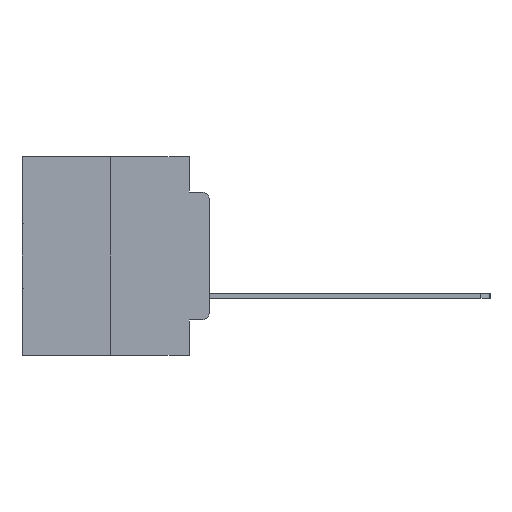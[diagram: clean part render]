
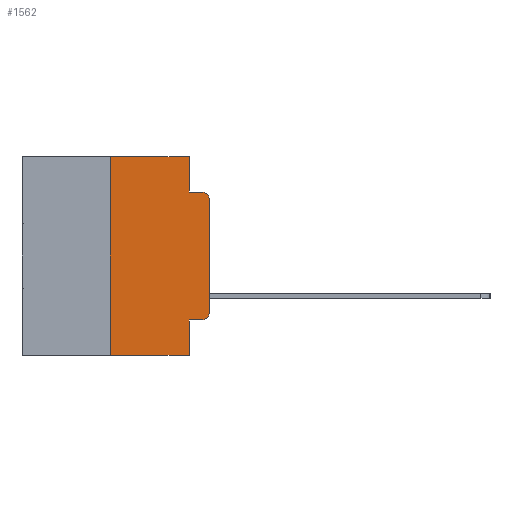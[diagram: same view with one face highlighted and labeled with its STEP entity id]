
A CAD part, left-side view. The second image highlights one B-rep face of the part: STEP entity #1562.
In plain terms, the highlighted planar face has unit normal (-1, 0, 0).
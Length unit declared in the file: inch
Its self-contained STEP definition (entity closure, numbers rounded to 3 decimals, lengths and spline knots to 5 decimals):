
#157 = VERTEX_POINT ( 'NONE', #6908 ) ;
#313 = CARTESIAN_POINT ( 'NONE',  ( 0., 0.473, 0. ) ) ;
#1015 = DIRECTION ( 'NONE',  ( -1., 0., 0. ) ) ;
#1311 = EDGE_CURVE ( 'NONE', #157, #25976, #9049, .T. ) ;
#1342 = ORIENTED_EDGE ( 'NONE', *, *, #24308, .F. ) ;
#1346 = EDGE_LOOP ( 'NONE', ( #4672, #28072, #5410, #11544, #18711, #1342, #20058, #2801, #9098, #3564 ) ) ;
#1423 = VECTOR ( 'NONE', #27654, 39.37008 ) ;
#1562 = ADVANCED_FACE ( 'NONE', ( #13211 ), #24217, .F. ) ;
#1711 = VECTOR ( 'NONE', #5330, 39.37008 ) ;
#1929 = DIRECTION ( 'NONE',  ( 0., 0., -1. ) ) ;
#2098 = CARTESIAN_POINT ( 'NONE',  ( 0., 0.25, 0. ) ) ;
#2108 = DIRECTION ( 'NONE',  ( 0., 0., -1. ) ) ;
#2547 = CARTESIAN_POINT ( 'NONE',  ( 0., 0., 0. ) ) ;
#2667 = VERTEX_POINT ( 'NONE', #3909 ) ;
#2801 = ORIENTED_EDGE ( 'NONE', *, *, #21455, .F. ) ;
#2845 = VECTOR ( 'NONE', #22708, 39.37008 ) ;
#2879 = EDGE_CURVE ( 'NONE', #5140, #157, #10006, .T. ) ;
#2929 = CARTESIAN_POINT ( 'NONE',  ( 0., 0.051, 0. ) ) ;
#3564 = ORIENTED_EDGE ( 'NONE', *, *, #17172, .T. ) ;
#3574 = CARTESIAN_POINT ( 'NONE',  ( 0., 0.02, -0.1085 ) ) ;
#3793 = VECTOR ( 'NONE', #22663, 39.37008 ) ;
#3909 = CARTESIAN_POINT ( 'NONE',  ( 0., 0.051, 0. ) ) ;
#3998 = LINE ( 'NONE', #6684, #21099 ) ;
#4391 = CARTESIAN_POINT ( 'NONE',  ( 0., 0.473, 0. ) ) ;
#4672 = ORIENTED_EDGE ( 'NONE', *, *, #2879, .T. ) ;
#5140 = VERTEX_POINT ( 'NONE', #11904 ) ;
#5330 = DIRECTION ( 'NONE',  ( 0., 0., -1. ) ) ;
#5410 = ORIENTED_EDGE ( 'NONE', *, *, #28629, .F. ) ;
#5966 = DIRECTION ( 'NONE',  ( 0., 0., -1. ) ) ;
#6523 = CARTESIAN_POINT ( 'NONE',  ( 0., 0.051, -0.4115 ) ) ;
#6684 = CARTESIAN_POINT ( 'NONE',  ( 0., 0.051, -0.0885 ) ) ;
#6908 = CARTESIAN_POINT ( 'NONE',  ( 0., 0., -0.1085 ) ) ;
#7549 = VERTEX_POINT ( 'NONE', #21760 ) ;
#7624 = CARTESIAN_POINT ( 'NONE',  ( 0., 0.051, -0.0885 ) ) ;
#7722 = LINE ( 'NONE', #21300, #1423 ) ;
#7900 = VERTEX_POINT ( 'NONE', #7624 ) ;
#9014 = DIRECTION ( 'NONE',  ( 0., -1., 0. ) ) ;
#9049 = CIRCLE ( 'NONE', #26088, 0.02 ) ;
#9098 = ORIENTED_EDGE ( 'NONE', *, *, #18599, .T. ) ;
#9133 = LINE ( 'NONE', #313, #2845 ) ;
#9150 = VERTEX_POINT ( 'NONE', #16626 ) ;
#9151 = CIRCLE ( 'NONE', #21629, 0.02 ) ;
#9981 = VECTOR ( 'NONE', #1929, 39.37008 ) ;
#10006 = LINE ( 'NONE', #2547, #3793 ) ;
#10782 = CARTESIAN_POINT ( 'NONE',  ( 0., 0.02, -0.0885 ) ) ;
#11544 = ORIENTED_EDGE ( 'NONE', *, *, #25758, .F. ) ;
#11904 = CARTESIAN_POINT ( 'NONE',  ( 0., 0., -0.3915 ) ) ;
#13035 = LINE ( 'NONE', #2098, #24494 ) ;
#13211 = FACE_OUTER_BOUND ( 'NONE', #1346, .T. ) ;
#13247 = CARTESIAN_POINT ( 'NONE',  ( 0., 0.25, -0.5 ) ) ;
#14809 = CARTESIAN_POINT ( 'NONE',  ( 0., 0.02, -0.3915 ) ) ;
#15200 = LINE ( 'NONE', #15665, #9981 ) ;
#15665 = CARTESIAN_POINT ( 'NONE',  ( 0., 0.051, 0. ) ) ;
#15827 = DIRECTION ( 'NONE',  ( 1., 0., 0. ) ) ;
#16626 = CARTESIAN_POINT ( 'NONE',  ( 0., 0.25, 0. ) ) ;
#16998 = DIRECTION ( 'NONE',  ( 0., 0., -1. ) ) ;
#17172 = EDGE_CURVE ( 'NONE', #25715, #5140, #9151, .T. ) ;
#17335 = VERTEX_POINT ( 'NONE', #17463 ) ;
#17463 = CARTESIAN_POINT ( 'NONE',  ( 0., 0.051, -0.5 ) ) ;
#17989 = DIRECTION ( 'NONE',  ( 0., 0., 1. ) ) ;
#18407 = AXIS2_PLACEMENT_3D ( 'NONE', #4391, #15827, #2108 ) ;
#18599 = EDGE_CURVE ( 'NONE', #7549, #25715, #20344, .T. ) ;
#18639 = CARTESIAN_POINT ( 'NONE',  ( 0., 0.02, -0.4115 ) ) ;
#18711 = ORIENTED_EDGE ( 'NONE', *, *, #28835, .F. ) ;
#19287 = DIRECTION ( 'NONE',  ( -1., 0., 0. ) ) ;
#19737 = LINE ( 'NONE', #2929, #1711 ) ;
#20058 = ORIENTED_EDGE ( 'NONE', *, *, #24685, .T. ) ;
#20344 = LINE ( 'NONE', #6523, #25365 ) ;
#20378 = VERTEX_POINT ( 'NONE', #13247 ) ;
#21099 = VECTOR ( 'NONE', #9014, 39.37008 ) ;
#21300 = CARTESIAN_POINT ( 'NONE',  ( 0., 0.473, -0.5 ) ) ;
#21455 = EDGE_CURVE ( 'NONE', #7549, #17335, #15200, .T. ) ;
#21629 = AXIS2_PLACEMENT_3D ( 'NONE', #14809, #1015, #16998 ) ;
#21760 = CARTESIAN_POINT ( 'NONE',  ( 0., 0.051, -0.4115 ) ) ;
#22663 = DIRECTION ( 'NONE',  ( 0., 0., 1. ) ) ;
#22708 = DIRECTION ( 'NONE',  ( 0., -1., 0. ) ) ;
#24076 = DIRECTION ( 'NONE',  ( 0., -1., 0. ) ) ;
#24217 = PLANE ( 'NONE',  #18407 ) ;
#24308 = EDGE_CURVE ( 'NONE', #20378, #9150, #13035, .T. ) ;
#24494 = VECTOR ( 'NONE', #17989, 39.37008 ) ;
#24685 = EDGE_CURVE ( 'NONE', #20378, #17335, #7722, .T. ) ;
#25365 = VECTOR ( 'NONE', #24076, 39.37008 ) ;
#25715 = VERTEX_POINT ( 'NONE', #18639 ) ;
#25758 = EDGE_CURVE ( 'NONE', #2667, #7900, #19737, .T. ) ;
#25976 = VERTEX_POINT ( 'NONE', #10782 ) ;
#26088 = AXIS2_PLACEMENT_3D ( 'NONE', #3574, #19287, #5966 ) ;
#27654 = DIRECTION ( 'NONE',  ( 0., -1., 0. ) ) ;
#28072 = ORIENTED_EDGE ( 'NONE', *, *, #1311, .T. ) ;
#28629 = EDGE_CURVE ( 'NONE', #7900, #25976, #3998, .T. ) ;
#28835 = EDGE_CURVE ( 'NONE', #9150, #2667, #9133, .T. ) ;
